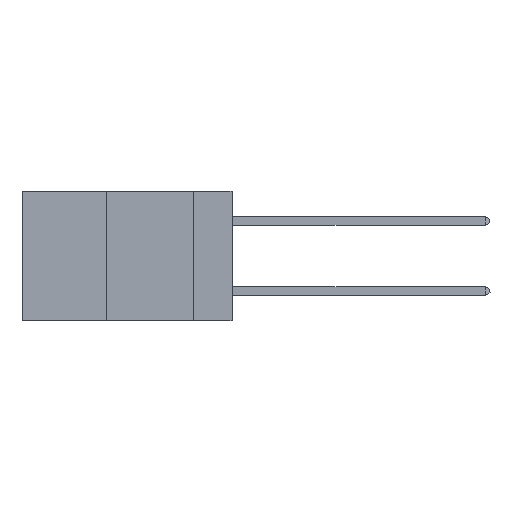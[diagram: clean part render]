
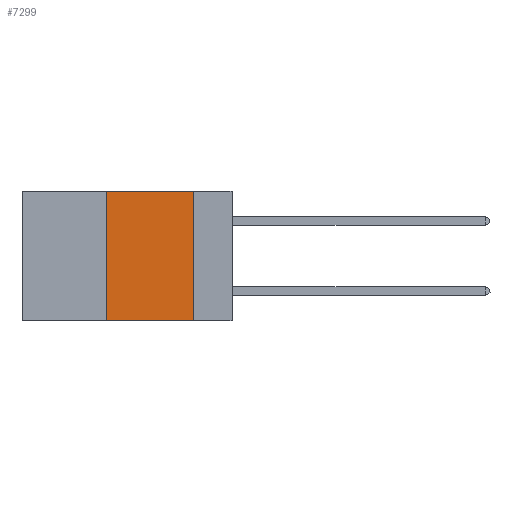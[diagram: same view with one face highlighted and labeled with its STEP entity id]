
A CAD part, left-side view. The second image highlights one B-rep face of the part: STEP entity #7299.
In plain terms, the highlighted planar face has unit normal (-1, 0, 0).
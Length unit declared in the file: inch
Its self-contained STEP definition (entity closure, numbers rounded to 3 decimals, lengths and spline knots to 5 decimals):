
#75 = EDGE_CURVE ( 'NONE', #6244, #3040, #8832, .T. ) ;
#565 = CARTESIAN_POINT ( 'NONE',  ( 0., 0.36, 0. ) ) ;
#1710 = AXIS2_PLACEMENT_3D ( 'NONE', #6562, #11460, #6453 ) ;
#2903 = VECTOR ( 'NONE', #4157, 39.37008 ) ;
#2973 = CARTESIAN_POINT ( 'NONE',  ( 0., 0.6, 0. ) ) ;
#3040 = VERTEX_POINT ( 'NONE', #6537 ) ;
#3274 = CARTESIAN_POINT ( 'NONE',  ( 0., 0.11, 0. ) ) ;
#3327 = CARTESIAN_POINT ( 'NONE',  ( 0., 0.36, -0.37 ) ) ;
#3572 = EDGE_CURVE ( 'NONE', #4597, #4517, #5029, .T. ) ;
#4157 = DIRECTION ( 'NONE',  ( 0., -1., 0. ) ) ;
#4411 = DIRECTION ( 'NONE',  ( 0., 0., 1. ) ) ;
#4517 = VERTEX_POINT ( 'NONE', #3274 ) ;
#4597 = VERTEX_POINT ( 'NONE', #7396 ) ;
#4872 = CARTESIAN_POINT ( 'NONE',  ( 0., 0.11, 0. ) ) ;
#5029 = LINE ( 'NONE', #2973, #2903 ) ;
#5200 = ORIENTED_EDGE ( 'NONE', *, *, #3572, .F. ) ;
#5368 = ORIENTED_EDGE ( 'NONE', *, *, #75, .T. ) ;
#5658 = DIRECTION ( 'NONE',  ( 0., 0., -1. ) ) ;
#5720 = LINE ( 'NONE', #4872, #12228 ) ;
#6244 = VERTEX_POINT ( 'NONE', #3327 ) ;
#6328 = LINE ( 'NONE', #565, #7642 ) ;
#6453 = DIRECTION ( 'NONE',  ( 0., 0., -1. ) ) ;
#6532 = EDGE_CURVE ( 'NONE', #4517, #3040, #5720, .T. ) ;
#6537 = CARTESIAN_POINT ( 'NONE',  ( 0., 0.11, -0.37 ) ) ;
#6562 = CARTESIAN_POINT ( 'NONE',  ( 0., 0.6, 0. ) ) ;
#6734 = ORIENTED_EDGE ( 'NONE', *, *, #6532, .F. ) ;
#7299 = ADVANCED_FACE ( 'NONE', ( #10202 ), #10383, .F. ) ;
#7396 = CARTESIAN_POINT ( 'NONE',  ( 0., 0.36, 0. ) ) ;
#7575 = EDGE_LOOP ( 'NONE', ( #6734, #5200, #9261, #5368 ) ) ;
#7642 = VECTOR ( 'NONE', #4411, 39.37008 ) ;
#7887 = CARTESIAN_POINT ( 'NONE',  ( 0., 0.6, -0.37 ) ) ;
#8655 = DIRECTION ( 'NONE',  ( 0., -1., 0. ) ) ;
#8832 = LINE ( 'NONE', #7887, #11955 ) ;
#9261 = ORIENTED_EDGE ( 'NONE', *, *, #12206, .F. ) ;
#10202 = FACE_OUTER_BOUND ( 'NONE', #7575, .T. ) ;
#10383 = PLANE ( 'NONE',  #1710 ) ;
#11460 = DIRECTION ( 'NONE',  ( 1., 0., 0. ) ) ;
#11955 = VECTOR ( 'NONE', #8655, 39.37008 ) ;
#12206 = EDGE_CURVE ( 'NONE', #6244, #4597, #6328, .T. ) ;
#12228 = VECTOR ( 'NONE', #5658, 39.37008 ) ;
